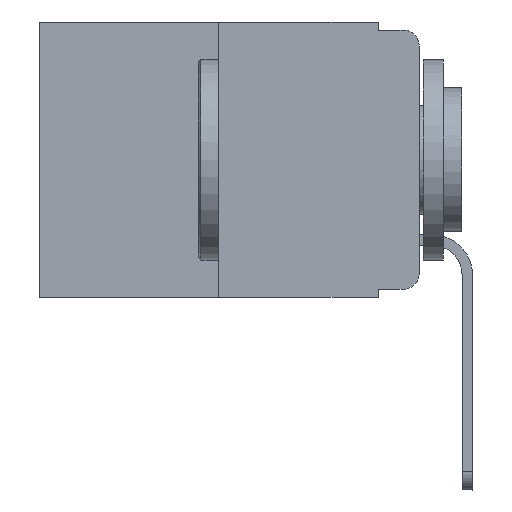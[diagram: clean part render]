
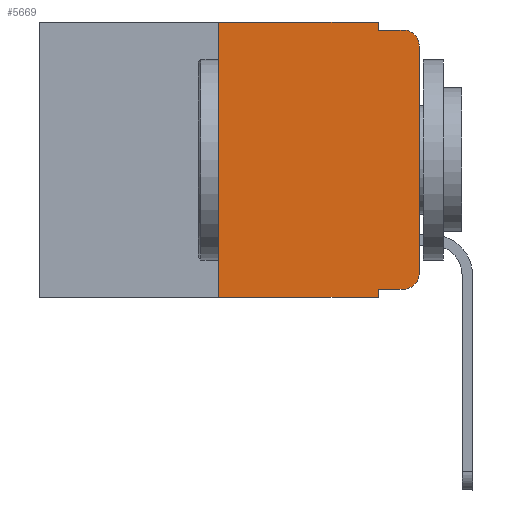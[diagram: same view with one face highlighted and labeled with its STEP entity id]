
A CAD part, left-side view. The second image highlights one B-rep face of the part: STEP entity #5669.
In plain terms, the highlighted planar face has unit normal (-1, 0, 0).
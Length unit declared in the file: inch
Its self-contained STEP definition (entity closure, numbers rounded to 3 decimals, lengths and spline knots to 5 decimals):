
#227 = DIRECTION ( 'NONE',  ( 0., 0., -1. ) ) ;
#256 = CARTESIAN_POINT ( 'NONE',  ( 0., 0., -0.313 ) ) ;
#351 = CARTESIAN_POINT ( 'NONE',  ( 0., 0.051, 0. ) ) ;
#447 = VERTEX_POINT ( 'NONE', #15038 ) ;
#452 = DIRECTION ( 'NONE',  ( -1., 0., 0. ) ) ;
#719 = VECTOR ( 'NONE', #17461, 39.37008 ) ;
#906 = CARTESIAN_POINT ( 'NONE',  ( 0., 0.051, -0.333 ) ) ;
#937 = VERTEX_POINT ( 'NONE', #17058 ) ;
#1736 = ORIENTED_EDGE ( 'NONE', *, *, #7487, .F. ) ;
#1761 = LINE ( 'NONE', #9604, #24058 ) ;
#1870 = DIRECTION ( 'NONE',  ( -1., 0., 0. ) ) ;
#2040 = FACE_OUTER_BOUND ( 'NONE', #15618, .T. ) ;
#3229 = CARTESIAN_POINT ( 'NONE',  ( 0., 0., 0. ) ) ;
#3439 = DIRECTION ( 'NONE',  ( 0., -1., 0. ) ) ;
#3478 = DIRECTION ( 'NONE',  ( 0., 0., 1. ) ) ;
#3605 = CARTESIAN_POINT ( 'NONE',  ( 0., 0.25, 0. ) ) ;
#4131 = CARTESIAN_POINT ( 'NONE',  ( 0., 0.051, -0.333 ) ) ;
#4392 = EDGE_CURVE ( 'NONE', #17518, #937, #19263, .T. ) ;
#4581 = ORIENTED_EDGE ( 'NONE', *, *, #4766, .T. ) ;
#4633 = DIRECTION ( 'NONE',  ( 0., -1., 0. ) ) ;
#4766 = EDGE_CURVE ( 'NONE', #24840, #10726, #10576, .T. ) ;
#4872 = EDGE_CURVE ( 'NONE', #11480, #24934, #8118, .T. ) ;
#5351 = ORIENTED_EDGE ( 'NONE', *, *, #14985, .T. ) ;
#5669 = ADVANCED_FACE ( 'NONE', ( #2040 ), #9871, .F. ) ;
#6327 = DIRECTION ( 'NONE',  ( 0., -1., 0. ) ) ;
#6425 = ORIENTED_EDGE ( 'NONE', *, *, #23330, .F. ) ;
#7408 = DIRECTION ( 'NONE',  ( 0., 0., -1. ) ) ;
#7487 = EDGE_CURVE ( 'NONE', #937, #447, #14376, .T. ) ;
#8118 = CIRCLE ( 'NONE', #15508, 0.02 ) ;
#8329 = DIRECTION ( 'NONE',  ( 0., 0., -1. ) ) ;
#8670 = EDGE_CURVE ( 'NONE', #19281, #17518, #11198, .T. ) ;
#9387 = AXIS2_PLACEMENT_3D ( 'NONE', #17730, #24294, #227 ) ;
#9500 = VERTEX_POINT ( 'NONE', #11750 ) ;
#9604 = CARTESIAN_POINT ( 'NONE',  ( 0., 0.051, -0.01 ) ) ;
#9871 = PLANE ( 'NONE',  #9387 ) ;
#10177 = LINE ( 'NONE', #15853, #17948 ) ;
#10541 = ORIENTED_EDGE ( 'NONE', *, *, #18494, .T. ) ;
#10576 = CIRCLE ( 'NONE', #14278, 0.02 ) ;
#10726 = VERTEX_POINT ( 'NONE', #11488 ) ;
#10988 = ORIENTED_EDGE ( 'NONE', *, *, #4392, .F. ) ;
#11198 = LINE ( 'NONE', #3605, #23881 ) ;
#11480 = VERTEX_POINT ( 'NONE', #16836 ) ;
#11488 = CARTESIAN_POINT ( 'NONE',  ( 0., 0.02, -0.01 ) ) ;
#11584 = CARTESIAN_POINT ( 'NONE',  ( 0., 0., -0.03 ) ) ;
#11750 = CARTESIAN_POINT ( 'NONE',  ( 0., 0.051, -0.343 ) ) ;
#11850 = LINE ( 'NONE', #4131, #14225 ) ;
#12318 = ORIENTED_EDGE ( 'NONE', *, *, #20938, .T. ) ;
#12404 = DIRECTION ( 'NONE',  ( 0., 0., -1. ) ) ;
#12469 = VECTOR ( 'NONE', #4633, 39.37008 ) ;
#12595 = CARTESIAN_POINT ( 'NONE',  ( 0., 0.473, -0.343 ) ) ;
#12607 = ORIENTED_EDGE ( 'NONE', *, *, #8670, .F. ) ;
#13958 = CARTESIAN_POINT ( 'NONE',  ( 0., 0.02, -0.313 ) ) ;
#14189 = CARTESIAN_POINT ( 'NONE',  ( 0., 0.25, -0.343 ) ) ;
#14225 = VECTOR ( 'NONE', #6327, 39.37008 ) ;
#14278 = AXIS2_PLACEMENT_3D ( 'NONE', #21172, #1870, #7408 ) ;
#14376 = LINE ( 'NONE', #351, #14741 ) ;
#14741 = VECTOR ( 'NONE', #8329, 39.37008 ) ;
#14985 = EDGE_CURVE ( 'NONE', #24934, #24840, #15191, .T. ) ;
#15038 = CARTESIAN_POINT ( 'NONE',  ( 0., 0.051, -0.01 ) ) ;
#15191 = LINE ( 'NONE', #3229, #15272 ) ;
#15272 = VECTOR ( 'NONE', #3478, 39.37008 ) ;
#15508 = AXIS2_PLACEMENT_3D ( 'NONE', #13958, #452, #12404 ) ;
#15618 = EDGE_LOOP ( 'NONE', ( #5351, #4581, #22025, #1736, #10988, #12607, #10541, #6425, #12318, #17000 ) ) ;
#15853 = CARTESIAN_POINT ( 'NONE',  ( 0., 0.051, 0. ) ) ;
#16836 = CARTESIAN_POINT ( 'NONE',  ( 0., 0.02, -0.333 ) ) ;
#17000 = ORIENTED_EDGE ( 'NONE', *, *, #4872, .T. ) ;
#17058 = CARTESIAN_POINT ( 'NONE',  ( 0., 0.051, 0. ) ) ;
#17283 = CARTESIAN_POINT ( 'NONE',  ( 0., 0.25, 0. ) ) ;
#17336 = CARTESIAN_POINT ( 'NONE',  ( 0., 0.473, 0. ) ) ;
#17461 = DIRECTION ( 'NONE',  ( 0., -1., 0. ) ) ;
#17518 = VERTEX_POINT ( 'NONE', #17283 ) ;
#17730 = CARTESIAN_POINT ( 'NONE',  ( 0., 0.473, 0. ) ) ;
#17948 = VECTOR ( 'NONE', #20219, 39.37008 ) ;
#18494 = EDGE_CURVE ( 'NONE', #19281, #9500, #24571, .T. ) ;
#19263 = LINE ( 'NONE', #17336, #719 ) ;
#19281 = VERTEX_POINT ( 'NONE', #14189 ) ;
#20219 = DIRECTION ( 'NONE',  ( 0., 0., -1. ) ) ;
#20938 = EDGE_CURVE ( 'NONE', #21134, #11480, #11850, .T. ) ;
#21134 = VERTEX_POINT ( 'NONE', #906 ) ;
#21172 = CARTESIAN_POINT ( 'NONE',  ( 0., 0.02, -0.03 ) ) ;
#21728 = EDGE_CURVE ( 'NONE', #447, #10726, #1761, .T. ) ;
#22025 = ORIENTED_EDGE ( 'NONE', *, *, #21728, .F. ) ;
#23042 = DIRECTION ( 'NONE',  ( 0., 0., 1. ) ) ;
#23330 = EDGE_CURVE ( 'NONE', #21134, #9500, #10177, .T. ) ;
#23881 = VECTOR ( 'NONE', #23042, 39.37008 ) ;
#24058 = VECTOR ( 'NONE', #3439, 39.37008 ) ;
#24294 = DIRECTION ( 'NONE',  ( 1., 0., 0. ) ) ;
#24571 = LINE ( 'NONE', #12595, #12469 ) ;
#24840 = VERTEX_POINT ( 'NONE', #11584 ) ;
#24934 = VERTEX_POINT ( 'NONE', #256 ) ;
